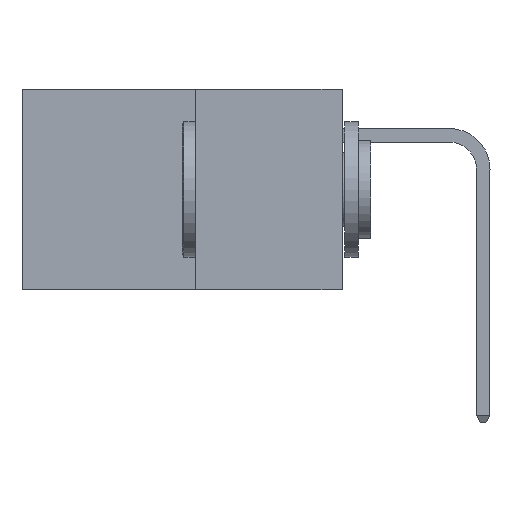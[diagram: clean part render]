
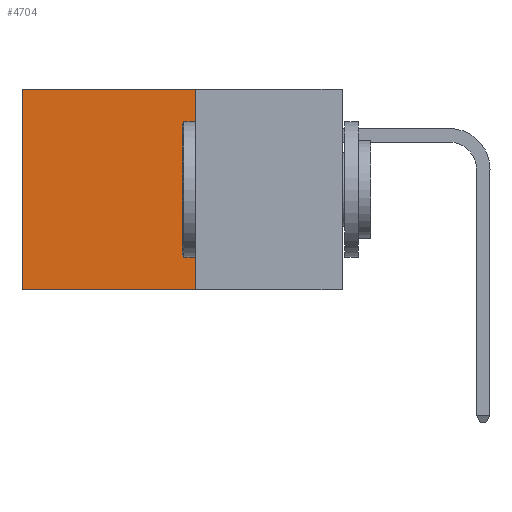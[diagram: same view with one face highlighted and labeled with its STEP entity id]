
A CAD part, left-side view. The second image highlights one B-rep face of the part: STEP entity #4704.
In plain terms, the highlighted planar face has unit normal (-1, 0, 0).
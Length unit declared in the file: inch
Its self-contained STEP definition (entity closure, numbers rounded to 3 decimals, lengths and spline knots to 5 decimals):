
#17 = DIRECTION ( 'NONE',  ( 1., 0., 0. ) ) ;
#157 = DIRECTION ( 'NONE',  ( 0., 0., -1. ) ) ;
#561 = VERTEX_POINT ( 'NONE', #5499 ) ;
#1057 = CARTESIAN_POINT ( 'NONE',  ( 0.277, 0.59, 0. ) ) ;
#1088 = DIRECTION ( 'NONE',  ( 0., 1., 0. ) ) ;
#1247 = ORIENTED_EDGE ( 'NONE', *, *, #6549, .T. ) ;
#1290 = ORIENTED_EDGE ( 'NONE', *, *, #3947, .F. ) ;
#1301 = ORIENTED_EDGE ( 'NONE', *, *, #7854, .F. ) ;
#1353 = ORIENTED_EDGE ( 'NONE', *, *, #5031, .T. ) ;
#1789 = VERTEX_POINT ( 'NONE', #9427 ) ;
#2637 = VECTOR ( 'NONE', #4913, 39.37008 ) ;
#2981 = CARTESIAN_POINT ( 'NONE',  ( 0.277, 0.59, -0.37 ) ) ;
#3947 = EDGE_CURVE ( 'NONE', #561, #9387, #10459, .T. ) ;
#4704 = ADVANCED_FACE ( 'NONE', ( #11169 ), #7276, .F. ) ;
#4913 = DIRECTION ( 'NONE',  ( 0., 0., -1. ) ) ;
#4962 = CARTESIAN_POINT ( 'NONE',  ( 0.277, 0.59, -0.37 ) ) ;
#5031 = EDGE_CURVE ( 'NONE', #1789, #8813, #8014, .T. ) ;
#5499 = CARTESIAN_POINT ( 'NONE',  ( 0.277, 0.27, -0.37 ) ) ;
#5882 = LINE ( 'NONE', #10388, #7876 ) ;
#6176 = DIRECTION ( 'NONE',  ( 0., 0., -1. ) ) ;
#6345 = AXIS2_PLACEMENT_3D ( 'NONE', #7756, #17, #157 ) ;
#6478 = VECTOR ( 'NONE', #1088, 39.37008 ) ;
#6549 = EDGE_CURVE ( 'NONE', #8813, #9387, #9725, .T. ) ;
#7029 = CARTESIAN_POINT ( 'NONE',  ( 0.277, 0.27, -0.37 ) ) ;
#7127 = DIRECTION ( 'NONE',  ( 0., 1., 0. ) ) ;
#7276 = PLANE ( 'NONE',  #6345 ) ;
#7589 = CARTESIAN_POINT ( 'NONE',  ( 0.277, 0.27, 0. ) ) ;
#7756 = CARTESIAN_POINT ( 'NONE',  ( 0.277, 0.27, -0.37 ) ) ;
#7854 = EDGE_CURVE ( 'NONE', #1789, #561, #5882, .T. ) ;
#7876 = VECTOR ( 'NONE', #6176, 39.37008 ) ;
#8014 = LINE ( 'NONE', #7589, #10255 ) ;
#8711 = EDGE_LOOP ( 'NONE', ( #1247, #1290, #1301, #1353 ) ) ;
#8813 = VERTEX_POINT ( 'NONE', #1057 ) ;
#9387 = VERTEX_POINT ( 'NONE', #2981 ) ;
#9427 = CARTESIAN_POINT ( 'NONE',  ( 0.277, 0.27, 0. ) ) ;
#9725 = LINE ( 'NONE', #4962, #2637 ) ;
#10255 = VECTOR ( 'NONE', #7127, 39.37008 ) ;
#10388 = CARTESIAN_POINT ( 'NONE',  ( 0.277, 0.27, -0.37 ) ) ;
#10459 = LINE ( 'NONE', #7029, #6478 ) ;
#11169 = FACE_OUTER_BOUND ( 'NONE', #8711, .T. ) ;
